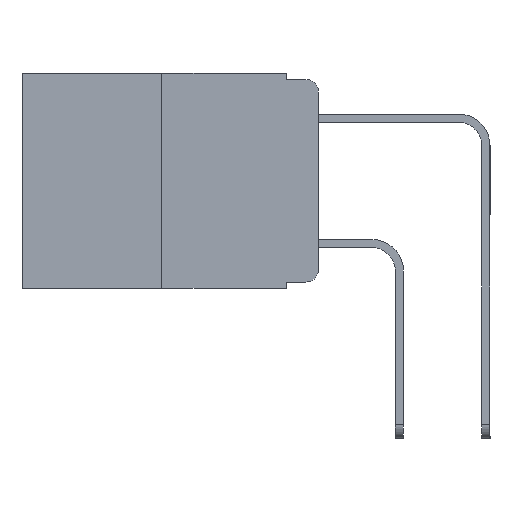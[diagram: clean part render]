
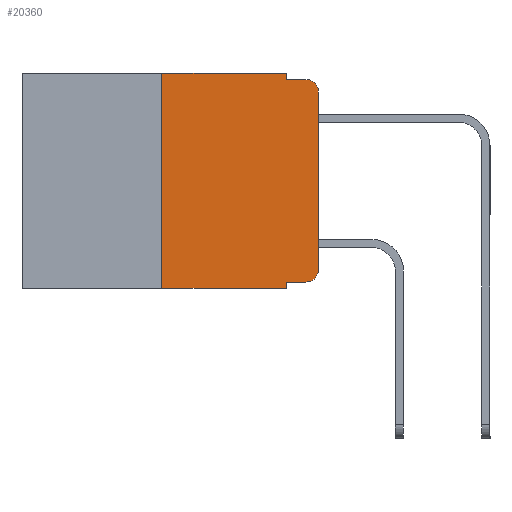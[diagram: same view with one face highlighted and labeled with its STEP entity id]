
A CAD part, left-side view. The second image highlights one B-rep face of the part: STEP entity #20360.
In plain terms, the highlighted planar face has unit normal (-1, 0, 0).
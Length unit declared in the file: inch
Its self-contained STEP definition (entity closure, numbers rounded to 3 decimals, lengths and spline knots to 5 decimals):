
#70 = EDGE_CURVE ( 'NONE', #18108, #166, #6575, .T. ) ;
#166 = VERTEX_POINT ( 'NONE', #21663 ) ;
#489 = CARTESIAN_POINT ( 'NONE',  ( 0., 0., 0. ) ) ;
#913 = ORIENTED_EDGE ( 'NONE', *, *, #14841, .F. ) ;
#1267 = CARTESIAN_POINT ( 'NONE',  ( 0., 0.25, 0. ) ) ;
#1380 = DIRECTION ( 'NONE',  ( 0., 0., -1. ) ) ;
#1382 = CIRCLE ( 'NONE', #7015, 0.02 ) ;
#1901 = CARTESIAN_POINT ( 'NONE',  ( 0., 0.051, -0.01 ) ) ;
#2153 = PLANE ( 'NONE',  #5710 ) ;
#2512 = AXIS2_PLACEMENT_3D ( 'NONE', #22331, #12055, #1380 ) ;
#2897 = ORIENTED_EDGE ( 'NONE', *, *, #15260, .F. ) ;
#3440 = LINE ( 'NONE', #5543, #21457 ) ;
#3658 = DIRECTION ( 'NONE',  ( 0., 0., -1. ) ) ;
#4000 = DIRECTION ( 'NONE',  ( 0., 0., -1. ) ) ;
#4343 = ORIENTED_EDGE ( 'NONE', *, *, #17472, .T. ) ;
#5496 = DIRECTION ( 'NONE',  ( -1., 0., 0. ) ) ;
#5543 = CARTESIAN_POINT ( 'NONE',  ( 0., 0.25, 0. ) ) ;
#5625 = VERTEX_POINT ( 'NONE', #13841 ) ;
#5710 = AXIS2_PLACEMENT_3D ( 'NONE', #7545, #14537, #4000 ) ;
#5745 = ORIENTED_EDGE ( 'NONE', *, *, #10229, .F. ) ;
#6575 = LINE ( 'NONE', #489, #19318 ) ;
#6888 = ORIENTED_EDGE ( 'NONE', *, *, #16146, .F. ) ;
#7015 = AXIS2_PLACEMENT_3D ( 'NONE', #15941, #5496, #17694 ) ;
#7350 = EDGE_CURVE ( 'NONE', #16696, #13601, #19875, .T. ) ;
#7545 = CARTESIAN_POINT ( 'NONE',  ( 0., 0.473, 0. ) ) ;
#7606 = LINE ( 'NONE', #7757, #11691 ) ;
#7690 = ORIENTED_EDGE ( 'NONE', *, *, #17278, .T. ) ;
#7697 = VERTEX_POINT ( 'NONE', #19766 ) ;
#7757 = CARTESIAN_POINT ( 'NONE',  ( 0., 0.051, -0.333 ) ) ;
#8072 = CARTESIAN_POINT ( 'NONE',  ( 0., 0.02, -0.333 ) ) ;
#8320 = CIRCLE ( 'NONE', #2512, 0.02 ) ;
#8702 = LINE ( 'NONE', #20607, #11700 ) ;
#8744 = VECTOR ( 'NONE', #11824, 39.37008 ) ;
#9217 = LINE ( 'NONE', #21039, #13282 ) ;
#9800 = EDGE_LOOP ( 'NONE', ( #15284, #7690, #13398, #5745, #2897, #913, #20141, #6888, #4343, #14257 ) ) ;
#10229 = EDGE_CURVE ( 'NONE', #7697, #14237, #9217, .T. ) ;
#10877 = DIRECTION ( 'NONE',  ( 0., 0., 1. ) ) ;
#11315 = CARTESIAN_POINT ( 'NONE',  ( 0., 0., -0.313 ) ) ;
#11469 = VERTEX_POINT ( 'NONE', #18041 ) ;
#11691 = VECTOR ( 'NONE', #14674, 39.37008 ) ;
#11700 = VECTOR ( 'NONE', #12029, 39.37008 ) ;
#11824 = DIRECTION ( 'NONE',  ( 0., -1., 0. ) ) ;
#12029 = DIRECTION ( 'NONE',  ( 0., 0., -1. ) ) ;
#12055 = DIRECTION ( 'NONE',  ( -1., 0., 0. ) ) ;
#12900 = EDGE_CURVE ( 'NONE', #16012, #18108, #8320, .T. ) ;
#13282 = VECTOR ( 'NONE', #3658, 39.37008 ) ;
#13357 = VERTEX_POINT ( 'NONE', #1267 ) ;
#13370 = LINE ( 'NONE', #16955, #8744 ) ;
#13398 = ORIENTED_EDGE ( 'NONE', *, *, #16285, .F. ) ;
#13540 = DIRECTION ( 'NONE',  ( 0., -1., 0. ) ) ;
#13601 = VERTEX_POINT ( 'NONE', #14301 ) ;
#13841 = CARTESIAN_POINT ( 'NONE',  ( 0., 0.051, -0.333 ) ) ;
#14129 = LINE ( 'NONE', #17599, #22714 ) ;
#14237 = VERTEX_POINT ( 'NONE', #1901 ) ;
#14257 = ORIENTED_EDGE ( 'NONE', *, *, #12900, .T. ) ;
#14301 = CARTESIAN_POINT ( 'NONE',  ( 0., 0.051, -0.343 ) ) ;
#14537 = DIRECTION ( 'NONE',  ( 1., 0., 0. ) ) ;
#14674 = DIRECTION ( 'NONE',  ( 0., -1., 0. ) ) ;
#14841 = EDGE_CURVE ( 'NONE', #16696, #13357, #3440, .T. ) ;
#15260 = EDGE_CURVE ( 'NONE', #13357, #7697, #13370, .T. ) ;
#15284 = ORIENTED_EDGE ( 'NONE', *, *, #70, .T. ) ;
#15309 = VECTOR ( 'NONE', #13540, 39.37008 ) ;
#15941 = CARTESIAN_POINT ( 'NONE',  ( 0., 0.02, -0.03 ) ) ;
#16012 = VERTEX_POINT ( 'NONE', #8072 ) ;
#16146 = EDGE_CURVE ( 'NONE', #5625, #13601, #8702, .T. ) ;
#16285 = EDGE_CURVE ( 'NONE', #14237, #11469, #14129, .T. ) ;
#16494 = DIRECTION ( 'NONE',  ( 0., 0., 1. ) ) ;
#16696 = VERTEX_POINT ( 'NONE', #22122 ) ;
#16955 = CARTESIAN_POINT ( 'NONE',  ( 0., 0.473, 0. ) ) ;
#17008 = CARTESIAN_POINT ( 'NONE',  ( 0., 0.473, -0.343 ) ) ;
#17278 = EDGE_CURVE ( 'NONE', #166, #11469, #1382, .T. ) ;
#17472 = EDGE_CURVE ( 'NONE', #5625, #16012, #7606, .T. ) ;
#17599 = CARTESIAN_POINT ( 'NONE',  ( 0., 0.051, -0.01 ) ) ;
#17694 = DIRECTION ( 'NONE',  ( 0., 0., -1. ) ) ;
#17729 = FACE_OUTER_BOUND ( 'NONE', #9800, .T. ) ;
#18041 = CARTESIAN_POINT ( 'NONE',  ( 0., 0.02, -0.01 ) ) ;
#18108 = VERTEX_POINT ( 'NONE', #11315 ) ;
#19318 = VECTOR ( 'NONE', #16494, 39.37008 ) ;
#19320 = DIRECTION ( 'NONE',  ( 0., -1., 0. ) ) ;
#19766 = CARTESIAN_POINT ( 'NONE',  ( 0., 0.051, 0. ) ) ;
#19875 = LINE ( 'NONE', #17008, #15309 ) ;
#20141 = ORIENTED_EDGE ( 'NONE', *, *, #7350, .T. ) ;
#20360 = ADVANCED_FACE ( 'NONE', ( #17729 ), #2153, .F. ) ;
#20607 = CARTESIAN_POINT ( 'NONE',  ( 0., 0.051, 0. ) ) ;
#21039 = CARTESIAN_POINT ( 'NONE',  ( 0., 0.051, 0. ) ) ;
#21457 = VECTOR ( 'NONE', #10877, 39.37008 ) ;
#21663 = CARTESIAN_POINT ( 'NONE',  ( 0., 0., -0.03 ) ) ;
#22122 = CARTESIAN_POINT ( 'NONE',  ( 0., 0.25, -0.343 ) ) ;
#22331 = CARTESIAN_POINT ( 'NONE',  ( 0., 0.02, -0.313 ) ) ;
#22714 = VECTOR ( 'NONE', #19320, 39.37008 ) ;
